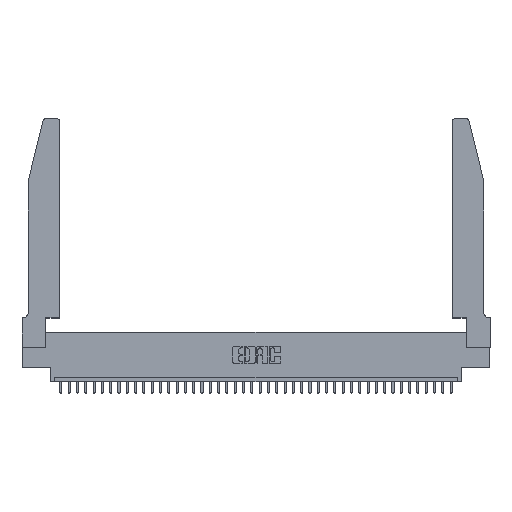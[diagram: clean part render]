
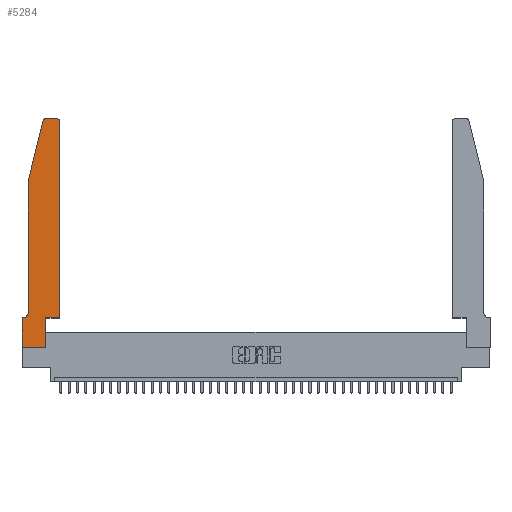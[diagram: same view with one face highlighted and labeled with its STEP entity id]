
A CAD part, top view. The second image highlights one B-rep face of the part: STEP entity #5284.
In plain terms, the highlighted planar face has unit normal (0, 0, 1).
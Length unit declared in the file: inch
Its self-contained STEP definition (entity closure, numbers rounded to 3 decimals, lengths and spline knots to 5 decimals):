
#175 = VERTEX_POINT ( 'NONE', #28486 ) ;
#679 = ORIENTED_EDGE ( 'NONE', *, *, #23679, .T. ) ;
#1529 = CARTESIAN_POINT ( 'NONE',  ( 0.2865, 0., 0.37 ) ) ;
#1793 = EDGE_CURVE ( 'NONE', #11242, #14190, #37915, .T. ) ;
#2279 = AXIS2_PLACEMENT_3D ( 'NONE', #30131, #39191, #28063 ) ;
#2856 = VERTEX_POINT ( 'NONE', #16690 ) ;
#2859 = DIRECTION ( 'NONE',  ( -1., 0., 0. ) ) ;
#2867 = EDGE_CURVE ( 'NONE', #13887, #35180, #8725, .T. ) ;
#3020 = VECTOR ( 'NONE', #22414, 39.37008 ) ;
#3100 = VERTEX_POINT ( 'NONE', #20989 ) ;
#3217 = VERTEX_POINT ( 'NONE', #18920 ) ;
#3447 = DIRECTION ( 'NONE',  ( 1., 0., 0. ) ) ;
#3684 = LINE ( 'NONE', #29597, #15870 ) ;
#4121 = ORIENTED_EDGE ( 'NONE', *, *, #23041, .T. ) ;
#4259 = DIRECTION ( 'NONE',  ( 1., 0., 0. ) ) ;
#4274 = CARTESIAN_POINT ( 'NONE',  ( 0.0755, 0.35, 0.37 ) ) ;
#4563 = VECTOR ( 'NONE', #32280, 39.37008 ) ;
#4675 = CARTESIAN_POINT ( 'NONE',  ( 0.2865, 0.35, 0.37 ) ) ;
#5122 = CARTESIAN_POINT ( 'NONE',  ( 0.4505, 0.35, 0.37 ) ) ;
#5284 = ADVANCED_FACE ( 'NONE', ( #20213 ), #31690, .T. ) ;
#5307 = DIRECTION ( 'NONE',  ( 0., -1., 0. ) ) ;
#5995 = LINE ( 'NONE', #27851, #17655 ) ;
#6214 = VERTEX_POINT ( 'NONE', #1529 ) ;
#6228 = ORIENTED_EDGE ( 'NONE', *, *, #26065, .T. ) ;
#7356 = CARTESIAN_POINT ( 'NONE',  ( 0., 0.35, 0.37 ) ) ;
#7607 = CARTESIAN_POINT ( 'NONE',  ( 0., 0., 0.37 ) ) ;
#8519 = VECTOR ( 'NONE', #30026, 39.37008 ) ;
#8578 = ORIENTED_EDGE ( 'NONE', *, *, #12896, .T. ) ;
#8725 = CIRCLE ( 'NONE', #2279, 0.03 ) ;
#9513 = LINE ( 'NONE', #28127, #31854 ) ;
#10729 = CARTESIAN_POINT ( 'NONE',  ( 0.284, 2.72, 0.37 ) ) ;
#11123 = AXIS2_PLACEMENT_3D ( 'NONE', #33790, #21836, #2859 ) ;
#11242 = VERTEX_POINT ( 'NONE', #4675 ) ;
#11274 = EDGE_CURVE ( 'NONE', #27654, #39608, #30009, .T. ) ;
#11482 = ORIENTED_EDGE ( 'NONE', *, *, #26590, .T. ) ;
#12200 = AXIS2_PLACEMENT_3D ( 'NONE', #31974, #38757, #37476 ) ;
#12896 = EDGE_CURVE ( 'NONE', #14190, #13887, #37554, .T. ) ;
#13887 = VERTEX_POINT ( 'NONE', #29110 ) ;
#14011 = EDGE_CURVE ( 'NONE', #6214, #11242, #5995, .T. ) ;
#14123 = ORIENTED_EDGE ( 'NONE', *, *, #11274, .T. ) ;
#14190 = VERTEX_POINT ( 'NONE', #5122 ) ;
#14530 = CIRCLE ( 'NONE', #26070, 0.03 ) ;
#15576 = CARTESIAN_POINT ( 'NONE',  ( 0.4505, 0.35, 0.37 ) ) ;
#15870 = VECTOR ( 'NONE', #5307, 39.37008 ) ;
#16202 = DIRECTION ( 'NONE',  ( 0., -1., 0. ) ) ;
#16690 = CARTESIAN_POINT ( 'NONE',  ( 0.0755, 2., 0.37 ) ) ;
#16909 = VECTOR ( 'NONE', #29235, 39.37008 ) ;
#17655 = VECTOR ( 'NONE', #30715, 39.37008 ) ;
#17838 = CARTESIAN_POINT ( 'NONE',  ( 0.0055, 0.35, 0.37 ) ) ;
#18236 = VECTOR ( 'NONE', #16202, 39.37008 ) ;
#18625 = EDGE_CURVE ( 'NONE', #35180, #3217, #32596, .T. ) ;
#18820 = ORIENTED_EDGE ( 'NONE', *, *, #1793, .T. ) ;
#18920 = CARTESIAN_POINT ( 'NONE',  ( 0.284, 2.75, 0.37 ) ) ;
#20213 = FACE_OUTER_BOUND ( 'NONE', #36302, .T. ) ;
#20256 = CARTESIAN_POINT ( 'NONE',  ( 0., 0., 0.37 ) ) ;
#20633 = EDGE_CURVE ( 'NONE', #3217, #3100, #14530, .T. ) ;
#20989 = CARTESIAN_POINT ( 'NONE',  ( 0.25487, 2.72718, 0.37 ) ) ;
#21083 = LINE ( 'NONE', #7607, #4563 ) ;
#21836 = DIRECTION ( 'NONE',  ( 0., 0., -1. ) ) ;
#22013 = CARTESIAN_POINT ( 'NONE',  ( 0., 0., 0.37 ) ) ;
#22264 = DIRECTION ( 'NONE',  ( -0.239, -0.971, 0. ) ) ;
#22414 = DIRECTION ( 'NONE',  ( -1., 0., 0. ) ) ;
#23041 = EDGE_CURVE ( 'NONE', #39608, #39783, #26496, .T. ) ;
#23679 = EDGE_CURVE ( 'NONE', #39783, #6214, #21083, .T. ) ;
#24045 = CARTESIAN_POINT ( 'NONE',  ( 0.4505, 0.35, 0.37 ) ) ;
#24533 = ORIENTED_EDGE ( 'NONE', *, *, #20633, .T. ) ;
#26065 = EDGE_CURVE ( 'NONE', #3100, #2856, #9513, .T. ) ;
#26070 = AXIS2_PLACEMENT_3D ( 'NONE', #10729, #35852, #4259 ) ;
#26496 = LINE ( 'NONE', #22013, #18236 ) ;
#26590 = EDGE_CURVE ( 'NONE', #175, #27654, #33293, .T. ) ;
#27654 = VERTEX_POINT ( 'NONE', #17838 ) ;
#27786 = VECTOR ( 'NONE', #3447, 39.37008 ) ;
#27851 = CARTESIAN_POINT ( 'NONE',  ( 0.2865, 0.35, 0.37 ) ) ;
#28063 = DIRECTION ( 'NONE',  ( 1., 0., 0. ) ) ;
#28127 = CARTESIAN_POINT ( 'NONE',  ( 0.0755, 2., 0.37 ) ) ;
#28486 = CARTESIAN_POINT ( 'NONE',  ( 0.0755, 0.42, 0.37 ) ) ;
#28923 = ORIENTED_EDGE ( 'NONE', *, *, #18625, .T. ) ;
#29110 = CARTESIAN_POINT ( 'NONE',  ( 0.4505, 2.72, 0.37 ) ) ;
#29235 = DIRECTION ( 'NONE',  ( -1., 0., 0. ) ) ;
#29597 = CARTESIAN_POINT ( 'NONE',  ( 0.0755, 2., 0.37 ) ) ;
#30009 = LINE ( 'NONE', #4274, #16909 ) ;
#30014 = ORIENTED_EDGE ( 'NONE', *, *, #14011, .T. ) ;
#30026 = DIRECTION ( 'NONE',  ( 0., 1., 0. ) ) ;
#30131 = CARTESIAN_POINT ( 'NONE',  ( 0.4205, 2.72, 0.37 ) ) ;
#30689 = ORIENTED_EDGE ( 'NONE', *, *, #2867, .T. ) ;
#30715 = DIRECTION ( 'NONE',  ( 0., 1., 0. ) ) ;
#31690 = PLANE ( 'NONE',  #12200 ) ;
#31854 = VECTOR ( 'NONE', #22264, 39.37008 ) ;
#31974 = CARTESIAN_POINT ( 'NONE',  ( 0., 0.35, 0.37 ) ) ;
#32280 = DIRECTION ( 'NONE',  ( 1., 0., 0. ) ) ;
#32596 = LINE ( 'NONE', #37451, #3020 ) ;
#33293 = CIRCLE ( 'NONE', #11123, 0.07 ) ;
#33790 = CARTESIAN_POINT ( 'NONE',  ( 0.0055, 0.42, 0.37 ) ) ;
#35180 = VERTEX_POINT ( 'NONE', #37901 ) ;
#35852 = DIRECTION ( 'NONE',  ( 0., 0., 1. ) ) ;
#35911 = ORIENTED_EDGE ( 'NONE', *, *, #36899, .T. ) ;
#36302 = EDGE_LOOP ( 'NONE', ( #28923, #24533, #6228, #35911, #11482, #14123, #4121, #679, #30014, #18820, #8578, #30689 ) ) ;
#36899 = EDGE_CURVE ( 'NONE', #2856, #175, #3684, .T. ) ;
#37451 = CARTESIAN_POINT ( 'NONE',  ( 0.2605, 2.75, 0.37 ) ) ;
#37476 = DIRECTION ( 'NONE',  ( 1., 0., 0. ) ) ;
#37554 = LINE ( 'NONE', #24045, #8519 ) ;
#37901 = CARTESIAN_POINT ( 'NONE',  ( 0.4205, 2.75, 0.37 ) ) ;
#37915 = LINE ( 'NONE', #15576, #27786 ) ;
#38757 = DIRECTION ( 'NONE',  ( 0., 0., 1. ) ) ;
#39191 = DIRECTION ( 'NONE',  ( 0., 0., 1. ) ) ;
#39608 = VERTEX_POINT ( 'NONE', #7356 ) ;
#39783 = VERTEX_POINT ( 'NONE', #20256 ) ;
